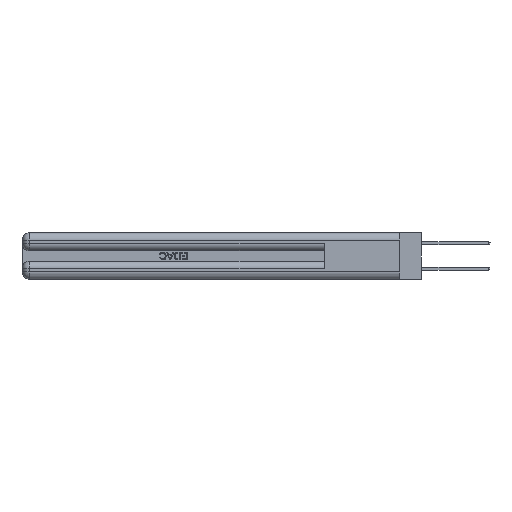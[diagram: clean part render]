
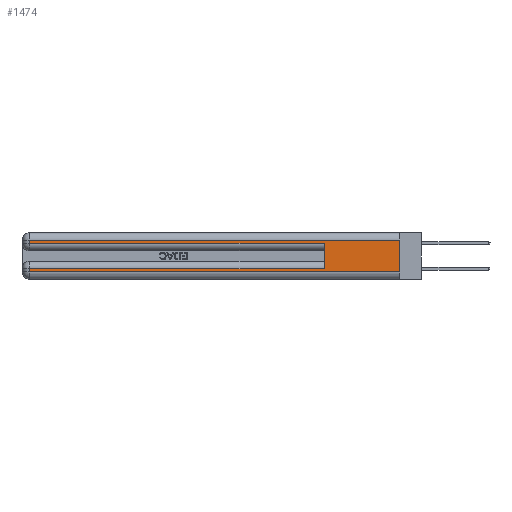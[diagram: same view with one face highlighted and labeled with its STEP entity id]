
A CAD part, left-side view. The second image highlights one B-rep face of the part: STEP entity #1474.
In plain terms, the highlighted planar face has unit normal (-1, 0, 0).
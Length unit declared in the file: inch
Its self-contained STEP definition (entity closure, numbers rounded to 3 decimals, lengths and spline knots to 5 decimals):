
#266 = DIRECTION ( 'NONE',  ( 0., -1., 0. ) ) ;
#1474 = ADVANCED_FACE ( 'NONE', ( #21970 ), #37696, .F. ) ;
#1685 = ORIENTED_EDGE ( 'NONE', *, *, #12337, .T. ) ;
#1710 = VERTEX_POINT ( 'NONE', #15110 ) ;
#1981 = EDGE_CURVE ( 'NONE', #42442, #13033, #3073, .T. ) ;
#2170 = EDGE_CURVE ( 'NONE', #47047, #13033, #31338, .T. ) ;
#2386 = EDGE_CURVE ( 'NONE', #42187, #5100, #24258, .T. ) ;
#3073 = LINE ( 'NONE', #41114, #17247 ) ;
#3291 = LINE ( 'NONE', #8448, #43297 ) ;
#4704 = VERTEX_POINT ( 'NONE', #29118 ) ;
#4817 = VECTOR ( 'NONE', #32748, 39.37008 ) ;
#5100 = VERTEX_POINT ( 'NONE', #14430 ) ;
#5410 = VECTOR ( 'NONE', #46811, 39.37008 ) ;
#5798 = DIRECTION ( 'NONE',  ( 0., 0., -1. ) ) ;
#6046 = DIRECTION ( 'NONE',  ( 0., 1., 0. ) ) ;
#8448 = CARTESIAN_POINT ( 'NONE',  ( 0., 2.94, 0.37 ) ) ;
#9835 = CARTESIAN_POINT ( 'NONE',  ( 0., 0., 0.37 ) ) ;
#12337 = EDGE_CURVE ( 'NONE', #4704, #5100, #14165, .T. ) ;
#12538 = VECTOR ( 'NONE', #20042, 39.37008 ) ;
#13033 = VERTEX_POINT ( 'NONE', #45444 ) ;
#13863 = CARTESIAN_POINT ( 'NONE',  ( 0., 2.94, 0.085 ) ) ;
#14165 = LINE ( 'NONE', #45340, #42361 ) ;
#14430 = CARTESIAN_POINT ( 'NONE',  ( 0., 0., 0.06 ) ) ;
#14598 = ORIENTED_EDGE ( 'NONE', *, *, #22589, .T. ) ;
#15110 = CARTESIAN_POINT ( 'NONE',  ( 0., 2.94, 0.31 ) ) ;
#15238 = CARTESIAN_POINT ( 'NONE',  ( 0., 0., 0.37 ) ) ;
#15326 = CARTESIAN_POINT ( 'NONE',  ( 0., 0., 0.31 ) ) ;
#15885 = EDGE_CURVE ( 'NONE', #1710, #47047, #3291, .T. ) ;
#17247 = VECTOR ( 'NONE', #42842, 39.37008 ) ;
#18070 = CARTESIAN_POINT ( 'NONE',  ( 0., 0.6, 0.085 ) ) ;
#18797 = DIRECTION ( 'NONE',  ( 0., 0., -1. ) ) ;
#20042 = DIRECTION ( 'NONE',  ( 0., 1., 0. ) ) ;
#20870 = CARTESIAN_POINT ( 'NONE',  ( 0., 0., 0.31 ) ) ;
#21358 = LINE ( 'NONE', #20870, #45460 ) ;
#21421 = ORIENTED_EDGE ( 'NONE', *, *, #30339, .T. ) ;
#21970 = FACE_OUTER_BOUND ( 'NONE', #42279, .T. ) ;
#22092 = CARTESIAN_POINT ( 'NONE',  ( 0., 2.94, 0.37 ) ) ;
#22490 = LINE ( 'NONE', #23671, #12538 ) ;
#22589 = EDGE_CURVE ( 'NONE', #42442, #38073, #22490, .T. ) ;
#22705 = ORIENTED_EDGE ( 'NONE', *, *, #2386, .F. ) ;
#23671 = CARTESIAN_POINT ( 'NONE',  ( 0., 0., 0.085 ) ) ;
#23706 = ORIENTED_EDGE ( 'NONE', *, *, #1981, .F. ) ;
#24258 = LINE ( 'NONE', #9835, #5410 ) ;
#24768 = CARTESIAN_POINT ( 'NONE',  ( 0., 2.94, 0.285 ) ) ;
#27330 = LINE ( 'NONE', #22092, #32048 ) ;
#28962 = CARTESIAN_POINT ( 'NONE',  ( 0., 0., 0.285 ) ) ;
#29118 = CARTESIAN_POINT ( 'NONE',  ( 0., 2.94, 0.06 ) ) ;
#29826 = ORIENTED_EDGE ( 'NONE', *, *, #15885, .T. ) ;
#30339 = EDGE_CURVE ( 'NONE', #42187, #1710, #21358, .T. ) ;
#31338 = LINE ( 'NONE', #28962, #4817 ) ;
#32048 = VECTOR ( 'NONE', #18797, 39.37008 ) ;
#32748 = DIRECTION ( 'NONE',  ( 0., -1., 0. ) ) ;
#34705 = ORIENTED_EDGE ( 'NONE', *, *, #2170, .T. ) ;
#37696 = PLANE ( 'NONE',  #45214 ) ;
#38073 = VERTEX_POINT ( 'NONE', #13863 ) ;
#41114 = CARTESIAN_POINT ( 'NONE',  ( 0., 0.6, 0.145 ) ) ;
#41476 = DIRECTION ( 'NONE',  ( 1., 0., 0. ) ) ;
#41732 = ORIENTED_EDGE ( 'NONE', *, *, #45318, .T. ) ;
#42187 = VERTEX_POINT ( 'NONE', #15326 ) ;
#42279 = EDGE_LOOP ( 'NONE', ( #22705, #21421, #29826, #34705, #23706, #14598, #41732, #1685 ) ) ;
#42361 = VECTOR ( 'NONE', #266, 39.37008 ) ;
#42442 = VERTEX_POINT ( 'NONE', #18070 ) ;
#42842 = DIRECTION ( 'NONE',  ( 0., 0., 1. ) ) ;
#43297 = VECTOR ( 'NONE', #5798, 39.37008 ) ;
#45214 = AXIS2_PLACEMENT_3D ( 'NONE', #15238, #41476, #45249 ) ;
#45249 = DIRECTION ( 'NONE',  ( 0., 0., -1. ) ) ;
#45318 = EDGE_CURVE ( 'NONE', #38073, #4704, #27330, .T. ) ;
#45340 = CARTESIAN_POINT ( 'NONE',  ( 0., 0., 0.06 ) ) ;
#45444 = CARTESIAN_POINT ( 'NONE',  ( 0., 0.6, 0.285 ) ) ;
#45460 = VECTOR ( 'NONE', #6046, 39.37008 ) ;
#46811 = DIRECTION ( 'NONE',  ( 0., 0., -1. ) ) ;
#47047 = VERTEX_POINT ( 'NONE', #24768 ) ;
